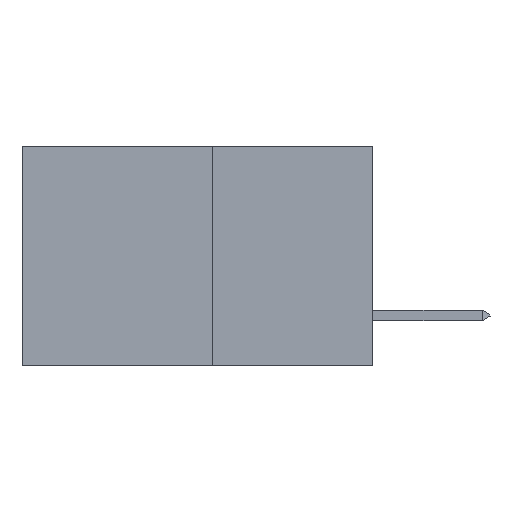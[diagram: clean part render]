
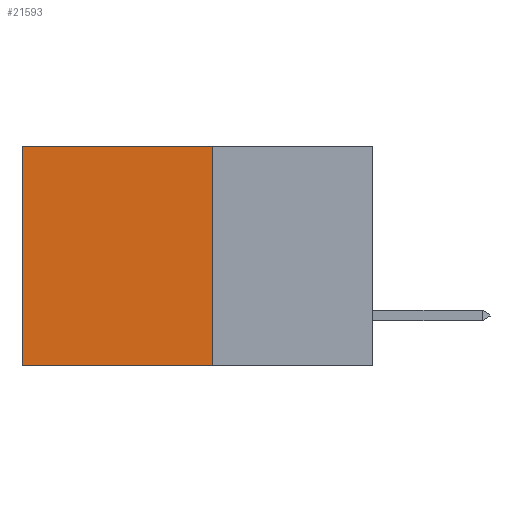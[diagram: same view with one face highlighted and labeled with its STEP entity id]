
A CAD part, left-side view. The second image highlights one B-rep face of the part: STEP entity #21593.
In plain terms, the highlighted planar face has unit normal (-1, 0, 0).
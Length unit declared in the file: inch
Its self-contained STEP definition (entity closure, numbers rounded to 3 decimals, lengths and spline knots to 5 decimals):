
#225 = ORIENTED_EDGE ( 'NONE', *, *, #8113, .T. ) ;
#1709 = VECTOR ( 'NONE', #10279, 39.37008 ) ;
#1849 = DIRECTION ( 'NONE',  ( 0., 0., -1. ) ) ;
#2199 = EDGE_LOOP ( 'NONE', ( #225, #8763, #25093, #24848 ) ) ;
#2966 = VERTEX_POINT ( 'NONE', #19422 ) ;
#3044 = LINE ( 'NONE', #24414, #1709 ) ;
#4534 = VECTOR ( 'NONE', #18966, 39.37008 ) ;
#4657 = FACE_OUTER_BOUND ( 'NONE', #2199, .T. ) ;
#5060 = CARTESIAN_POINT ( 'NONE',  ( 0.277, 0.59, -0.37 ) ) ;
#8113 = EDGE_CURVE ( 'NONE', #16303, #25949, #18978, .T. ) ;
#8276 = LINE ( 'NONE', #22162, #19103 ) ;
#8763 = ORIENTED_EDGE ( 'NONE', *, *, #8968, .F. ) ;
#8968 = EDGE_CURVE ( 'NONE', #24398, #25949, #16080, .T. ) ;
#10279 = DIRECTION ( 'NONE',  ( 0., 0., -1. ) ) ;
#11382 = EDGE_CURVE ( 'NONE', #2966, #16303, #8276, .T. ) ;
#12605 = CARTESIAN_POINT ( 'NONE',  ( 0.277, 0.27, -0.37 ) ) ;
#13602 = VECTOR ( 'NONE', #22538, 39.37008 ) ;
#14240 = DIRECTION ( 'NONE',  ( 1., 0., 0. ) ) ;
#14913 = CARTESIAN_POINT ( 'NONE',  ( 0.277, 0.27, -0.37 ) ) ;
#15233 = CARTESIAN_POINT ( 'NONE',  ( 0.277, 0.59, 0. ) ) ;
#15708 = EDGE_CURVE ( 'NONE', #2966, #24398, #3044, .T. ) ;
#16080 = LINE ( 'NONE', #14913, #4534 ) ;
#16303 = VERTEX_POINT ( 'NONE', #15233 ) ;
#18168 = DIRECTION ( 'NONE',  ( 0., 1., 0. ) ) ;
#18548 = CARTESIAN_POINT ( 'NONE',  ( 0.277, 0.59, -0.37 ) ) ;
#18966 = DIRECTION ( 'NONE',  ( 0., 1., 0. ) ) ;
#18978 = LINE ( 'NONE', #18548, #13602 ) ;
#19103 = VECTOR ( 'NONE', #18168, 39.37008 ) ;
#19422 = CARTESIAN_POINT ( 'NONE',  ( 0.277, 0.27, 0. ) ) ;
#20217 = PLANE ( 'NONE',  #20490 ) ;
#20490 = AXIS2_PLACEMENT_3D ( 'NONE', #26231, #14240, #1849 ) ;
#21593 = ADVANCED_FACE ( 'NONE', ( #4657 ), #20217, .F. ) ;
#22162 = CARTESIAN_POINT ( 'NONE',  ( 0.277, 0.27, 0. ) ) ;
#22538 = DIRECTION ( 'NONE',  ( 0., 0., -1. ) ) ;
#24398 = VERTEX_POINT ( 'NONE', #12605 ) ;
#24414 = CARTESIAN_POINT ( 'NONE',  ( 0.277, 0.27, -0.37 ) ) ;
#24848 = ORIENTED_EDGE ( 'NONE', *, *, #11382, .T. ) ;
#25093 = ORIENTED_EDGE ( 'NONE', *, *, #15708, .F. ) ;
#25949 = VERTEX_POINT ( 'NONE', #5060 ) ;
#26231 = CARTESIAN_POINT ( 'NONE',  ( 0.277, 0.27, -0.37 ) ) ;
